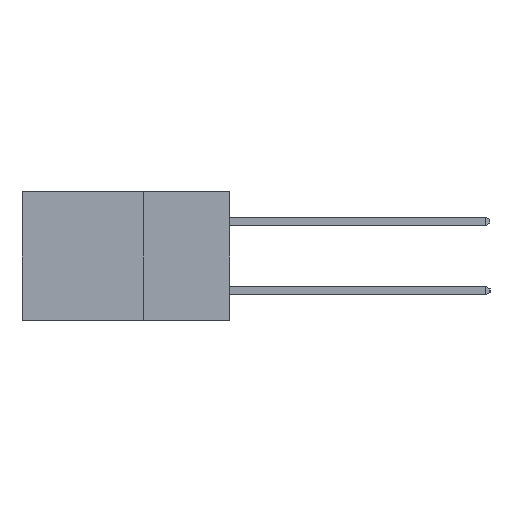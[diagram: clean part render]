
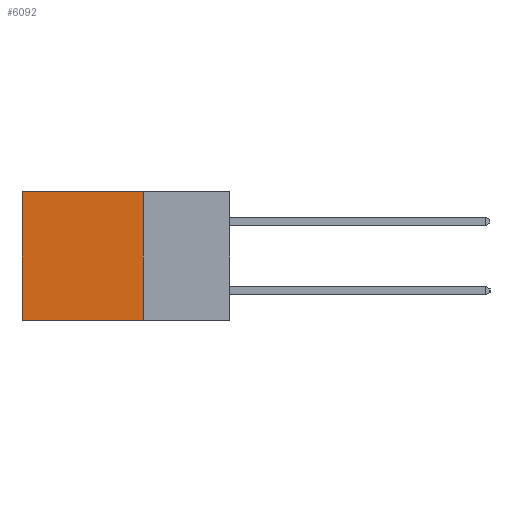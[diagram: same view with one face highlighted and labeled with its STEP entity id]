
A CAD part, left-side view. The second image highlights one B-rep face of the part: STEP entity #6092.
In plain terms, the highlighted planar face has unit normal (-1, 0, 0).
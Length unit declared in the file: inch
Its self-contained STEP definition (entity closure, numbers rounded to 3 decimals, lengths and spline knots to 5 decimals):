
#1642 = DIRECTION ( 'NONE',  ( 0., 1., 0. ) ) ;
#1857 = DIRECTION ( 'NONE',  ( 0., 0., -1. ) ) ;
#2250 = CARTESIAN_POINT ( 'NONE',  ( 0.2615, 0.25, -0.37 ) ) ;
#3705 = CARTESIAN_POINT ( 'NONE',  ( 0.2615, 0.6, -0.37 ) ) ;
#3752 = DIRECTION ( 'NONE',  ( 0., 0., -1. ) ) ;
#4709 = VECTOR ( 'NONE', #1642, 39.37008 ) ;
#4945 = FACE_OUTER_BOUND ( 'NONE', #18588, .T. ) ;
#6092 = ADVANCED_FACE ( 'NONE', ( #4945 ), #23969, .F. ) ;
#7102 = VERTEX_POINT ( 'NONE', #21232 ) ;
#7974 = LINE ( 'NONE', #23258, #23277 ) ;
#9192 = ORIENTED_EDGE ( 'NONE', *, *, #14578, .T. ) ;
#10403 = DIRECTION ( 'NONE',  ( 0., 0., -1. ) ) ;
#12071 = CARTESIAN_POINT ( 'NONE',  ( 0.2615, 0.25, -0.37 ) ) ;
#13458 = ORIENTED_EDGE ( 'NONE', *, *, #23131, .F. ) ;
#13813 = AXIS2_PLACEMENT_3D ( 'NONE', #12071, #14040, #1857 ) ;
#14040 = DIRECTION ( 'NONE',  ( 1., 0., 0. ) ) ;
#14568 = CARTESIAN_POINT ( 'NONE',  ( 0.2615, 0.6, 0. ) ) ;
#14578 = EDGE_CURVE ( 'NONE', #25011, #21953, #15996, .T. ) ;
#15236 = VECTOR ( 'NONE', #10403, 39.37008 ) ;
#15844 = CARTESIAN_POINT ( 'NONE',  ( 0.2615, 0.25, 0. ) ) ;
#15996 = LINE ( 'NONE', #16906, #25882 ) ;
#16089 = ORIENTED_EDGE ( 'NONE', *, *, #22179, .F. ) ;
#16114 = LINE ( 'NONE', #15844, #4709 ) ;
#16906 = CARTESIAN_POINT ( 'NONE',  ( 0.2615, 0.6, -0.37 ) ) ;
#18588 = EDGE_LOOP ( 'NONE', ( #9192, #13458, #16089, #21765 ) ) ;
#19415 = DIRECTION ( 'NONE',  ( 0., 1., 0. ) ) ;
#20921 = CARTESIAN_POINT ( 'NONE',  ( 0.2615, 0.25, 0. ) ) ;
#21232 = CARTESIAN_POINT ( 'NONE',  ( 0.2615, 0.25, -0.37 ) ) ;
#21765 = ORIENTED_EDGE ( 'NONE', *, *, #23274, .T. ) ;
#21781 = LINE ( 'NONE', #2250, #15236 ) ;
#21953 = VERTEX_POINT ( 'NONE', #3705 ) ;
#22179 = EDGE_CURVE ( 'NONE', #25132, #7102, #21781, .T. ) ;
#23131 = EDGE_CURVE ( 'NONE', #7102, #21953, #7974, .T. ) ;
#23258 = CARTESIAN_POINT ( 'NONE',  ( 0.2615, 0.25, -0.37 ) ) ;
#23274 = EDGE_CURVE ( 'NONE', #25132, #25011, #16114, .T. ) ;
#23277 = VECTOR ( 'NONE', #19415, 39.37008 ) ;
#23969 = PLANE ( 'NONE',  #13813 ) ;
#25011 = VERTEX_POINT ( 'NONE', #14568 ) ;
#25132 = VERTEX_POINT ( 'NONE', #20921 ) ;
#25882 = VECTOR ( 'NONE', #3752, 39.37008 ) ;
